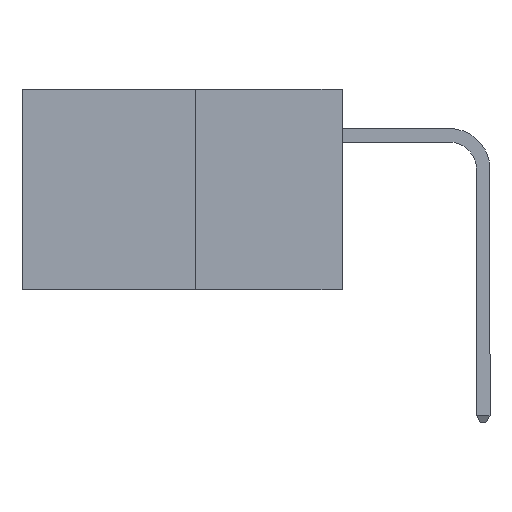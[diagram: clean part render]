
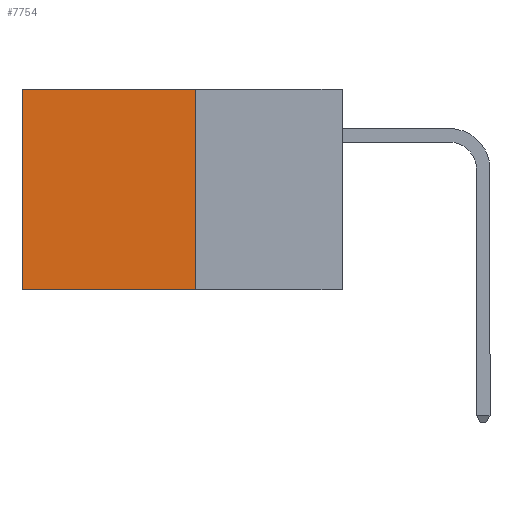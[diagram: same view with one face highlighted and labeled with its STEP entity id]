
A CAD part, left-side view. The second image highlights one B-rep face of the part: STEP entity #7754.
In plain terms, the highlighted planar face has unit normal (-1, 0, 0).
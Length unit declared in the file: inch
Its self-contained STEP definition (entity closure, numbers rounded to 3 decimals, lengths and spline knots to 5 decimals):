
#309 = VERTEX_POINT ( 'NONE', #8736 ) ;
#685 = LINE ( 'NONE', #1769, #17909 ) ;
#738 = CARTESIAN_POINT ( 'NONE',  ( 0.277, 0.27, -0.37 ) ) ;
#827 = DIRECTION ( 'NONE',  ( 0., 0., -1. ) ) ;
#1007 = EDGE_CURVE ( 'NONE', #21440, #9964, #1985, .T. ) ;
#1319 = ORIENTED_EDGE ( 'NONE', *, *, #20389, .T. ) ;
#1769 = CARTESIAN_POINT ( 'NONE',  ( 0.277, 0.59, -0.37 ) ) ;
#1985 = LINE ( 'NONE', #12970, #10416 ) ;
#2350 = CARTESIAN_POINT ( 'NONE',  ( 0.277, 0.59, 0. ) ) ;
#4546 = VECTOR ( 'NONE', #827, 39.37008 ) ;
#4763 = DIRECTION ( 'NONE',  ( 0., 1., 0. ) ) ;
#6034 = PLANE ( 'NONE',  #15277 ) ;
#6818 = DIRECTION ( 'NONE',  ( 0., 0., -1. ) ) ;
#6963 = EDGE_CURVE ( 'NONE', #309, #21440, #9089, .T. ) ;
#7754 = ADVANCED_FACE ( 'NONE', ( #11661 ), #6034, .F. ) ;
#8736 = CARTESIAN_POINT ( 'NONE',  ( 0.277, 0.27, 0. ) ) ;
#8869 = ORIENTED_EDGE ( 'NONE', *, *, #12934, .T. ) ;
#9089 = LINE ( 'NONE', #9163, #4546 ) ;
#9163 = CARTESIAN_POINT ( 'NONE',  ( 0.277, 0.27, -0.37 ) ) ;
#9296 = VECTOR ( 'NONE', #4763, 39.37008 ) ;
#9320 = EDGE_LOOP ( 'NONE', ( #8869, #12654, #12900, #1319 ) ) ;
#9506 = DIRECTION ( 'NONE',  ( 1., 0., 0. ) ) ;
#9964 = VERTEX_POINT ( 'NONE', #17712 ) ;
#10416 = VECTOR ( 'NONE', #16491, 39.37008 ) ;
#11512 = CARTESIAN_POINT ( 'NONE',  ( 0.277, 0.27, 0. ) ) ;
#11661 = FACE_OUTER_BOUND ( 'NONE', #9320, .T. ) ;
#12654 = ORIENTED_EDGE ( 'NONE', *, *, #1007, .F. ) ;
#12900 = ORIENTED_EDGE ( 'NONE', *, *, #6963, .F. ) ;
#12934 = EDGE_CURVE ( 'NONE', #15678, #9964, #685, .T. ) ;
#12970 = CARTESIAN_POINT ( 'NONE',  ( 0.277, 0.27, -0.37 ) ) ;
#13725 = LINE ( 'NONE', #11512, #9296 ) ;
#15277 = AXIS2_PLACEMENT_3D ( 'NONE', #19352, #9506, #21018 ) ;
#15678 = VERTEX_POINT ( 'NONE', #2350 ) ;
#16491 = DIRECTION ( 'NONE',  ( 0., 1., 0. ) ) ;
#17712 = CARTESIAN_POINT ( 'NONE',  ( 0.277, 0.59, -0.37 ) ) ;
#17909 = VECTOR ( 'NONE', #6818, 39.37008 ) ;
#19352 = CARTESIAN_POINT ( 'NONE',  ( 0.277, 0.27, -0.37 ) ) ;
#20389 = EDGE_CURVE ( 'NONE', #309, #15678, #13725, .T. ) ;
#21018 = DIRECTION ( 'NONE',  ( 0., 0., -1. ) ) ;
#21440 = VERTEX_POINT ( 'NONE', #738 ) ;
